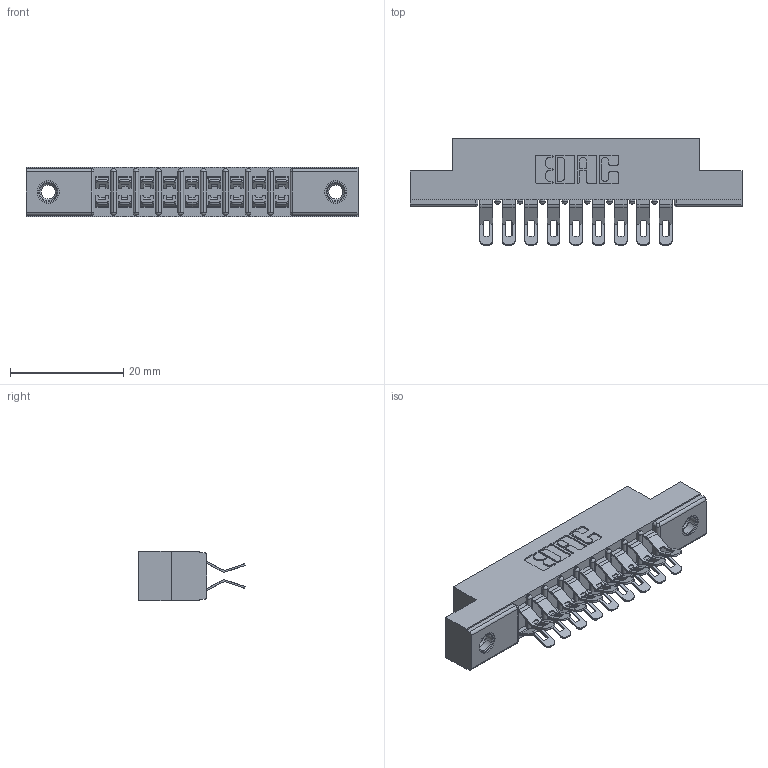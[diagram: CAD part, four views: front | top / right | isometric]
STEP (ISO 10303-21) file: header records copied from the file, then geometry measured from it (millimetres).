
FILE_DESCRIPTION (( 'STEP AP203' ), '1' );
FILE_NAME ('307-018-555-207.STEP', '2019-09-05T20:04:59', ( '' ), ( '' ), 'SwSTEP 2.0', 'SolidWorks 2016', '' );
FILE_SCHEMA (( 'CONFIG_CONTROL_DESIGN' ));
Length unit declared in the file: inch
Products named in the file (4): 307-290-001_555; 307 Part_.156 Dia Mounting Holes; 307-018-555-207; 345-250-001_345-250-005-103
Assembly tree (21 placements, depth 2):
  307-018-555-207
    307 Part_.156 Dia Mounting Holes
    307-290-001_555  x18
    345-250-001_345-250-005-103  x2
Bounding box: 58.67 x 18.75 x 8.71 mm (x, y, z)
Volume: 3879.5 mm3; surface area: 6508.5 mm2
Topology: 21 solids, 21 shells, 1286 faces, 3717 edges, 2418 vertices
Faces by surface type: plane 714, cylinder 536, sphere 20, cone 12, torus 4
Entity records: 13794 total; most frequent: CARTESIAN_POINT 2256, DIRECTION 2240, ORIENTED_EDGE 2228, EDGE_CURVE 1114, VECTOR 828, LINE 828, VERTEX_POINT 722, AXIS2_PLACEMENT_3D 706
